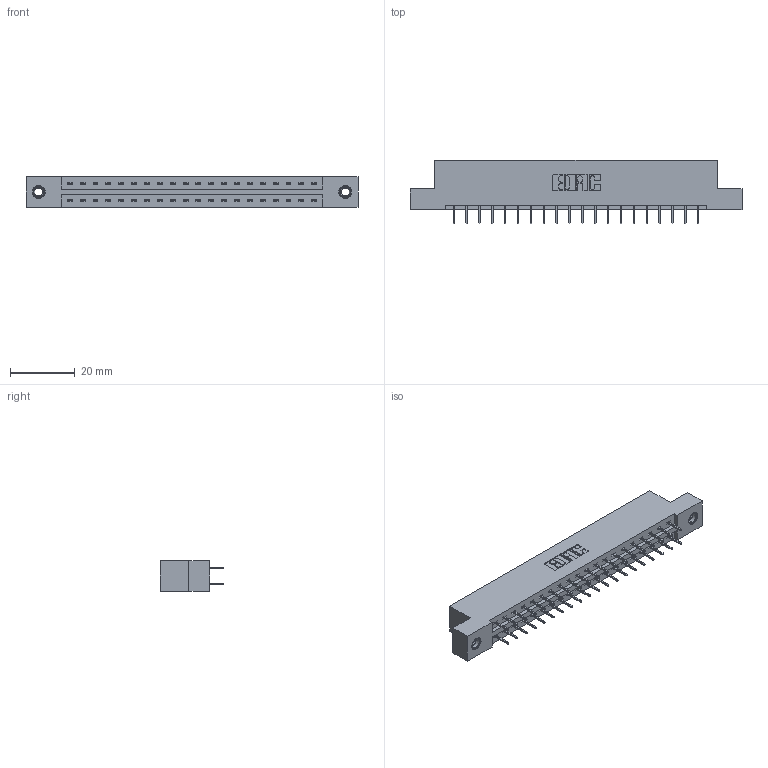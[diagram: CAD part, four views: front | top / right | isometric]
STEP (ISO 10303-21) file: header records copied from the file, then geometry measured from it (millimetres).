
FILE_DESCRIPTION (( 'STEP AP203' ), '1' );
FILE_NAME ('387-040-524-207.STEP', '2018-09-19T10:35:23', ( '' ), ( '' ), 'SwSTEP 2.0', 'SolidWorks 2016', '' );
FILE_SCHEMA (( 'CONFIG_CONTROL_DESIGN' ));
Length unit declared in the file: inch
Products named in the file (4): 337 Part_Flush Mounting Lugs - 0.156 Dia-TI; 345-292-001_345-293-124; 345-250-001_345-250-005-103; 387-040-524-207
Assembly tree (43 placements, depth 2):
  387-040-524-207
    337 Part_Flush Mounting Lugs - 0.156 Dia-TI
    345-292-001_345-293-124  x40
    345-250-001_345-250-005-103  x2
Bounding box: 102.26 x 19.69 x 9.4 mm (x, y, z)
Volume: 10410.1 mm3; surface area: 11403.4 mm2
Topology: 43 solids, 43 shells, 2494 faces, 7047 edges, 4530 vertices
Faces by surface type: plane 1862, cylinder 616, cone 12, torus 4
Entity records: 19612 total; most frequent: CARTESIAN_POINT 3301, ORIENTED_EDGE 3230, DIRECTION 2881, EDGE_CURVE 1615, VECTOR 1471, LINE 1471, VERTEX_POINT 1068, AXIS2_PLACEMENT_3D 705
